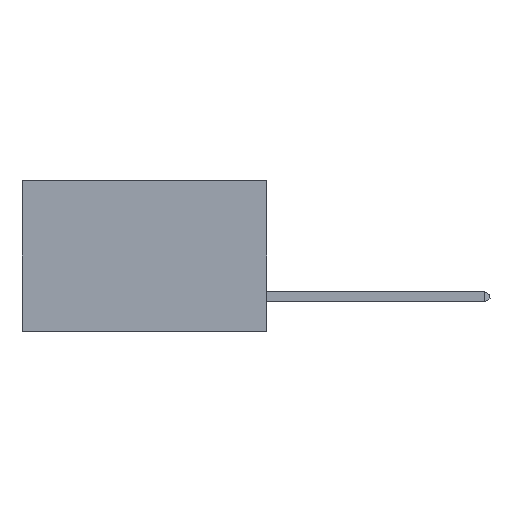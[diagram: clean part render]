
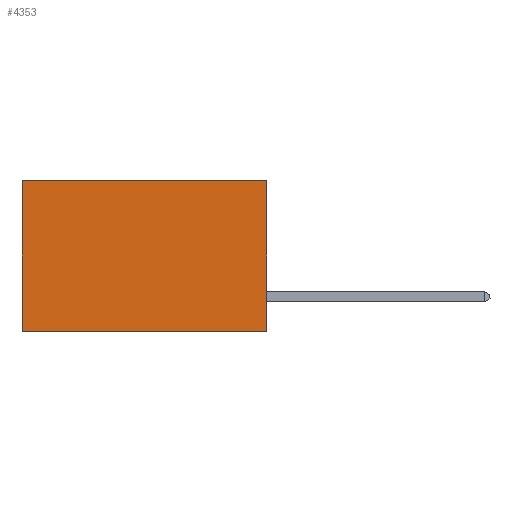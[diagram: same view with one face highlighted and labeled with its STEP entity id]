
A CAD part, left-side view. The second image highlights one B-rep face of the part: STEP entity #4353.
In plain terms, the highlighted planar face has unit normal (-1, 0, 0).
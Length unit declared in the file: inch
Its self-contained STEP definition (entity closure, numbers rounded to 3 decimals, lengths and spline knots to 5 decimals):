
#1136 = CARTESIAN_POINT ( 'NONE',  ( 0.2875, 0., 0. ) ) ;
#2256 = CARTESIAN_POINT ( 'NONE',  ( 0.2875, 0., 0. ) ) ;
#3129 = LINE ( 'NONE', #4401, #30596 ) ;
#3956 = LINE ( 'NONE', #25952, #26061 ) ;
#4353 = ADVANCED_FACE ( 'NONE', ( #4934 ), #23430, .F. ) ;
#4401 = CARTESIAN_POINT ( 'NONE',  ( 0.2875, 0., -0.37 ) ) ;
#4934 = FACE_OUTER_BOUND ( 'NONE', #14066, .T. ) ;
#5950 = DIRECTION ( 'NONE',  ( 1., 0., 0. ) ) ;
#6538 = DIRECTION ( 'NONE',  ( 0., 0., -1. ) ) ;
#8225 = EDGE_CURVE ( 'NONE', #13821, #19185, #3956, .T. ) ;
#9871 = VERTEX_POINT ( 'NONE', #10964 ) ;
#10056 = VERTEX_POINT ( 'NONE', #30152 ) ;
#10964 = CARTESIAN_POINT ( 'NONE',  ( 0.2875, 0., -0.37 ) ) ;
#11171 = VECTOR ( 'NONE', #6538, 39.37008 ) ;
#11800 = AXIS2_PLACEMENT_3D ( 'NONE', #29299, #5950, #22975 ) ;
#12745 = VECTOR ( 'NONE', #18794, 39.37008 ) ;
#13821 = VERTEX_POINT ( 'NONE', #2256 ) ;
#14066 = EDGE_LOOP ( 'NONE', ( #28393, #21594, #18133, #33533 ) ) ;
#16141 = CARTESIAN_POINT ( 'NONE',  ( 0.2875, 0.6, 0. ) ) ;
#18091 = DIRECTION ( 'NONE',  ( 0., 1., 0. ) ) ;
#18133 = ORIENTED_EDGE ( 'NONE', *, *, #21793, .F. ) ;
#18794 = DIRECTION ( 'NONE',  ( 0., 0., -1. ) ) ;
#19185 = VERTEX_POINT ( 'NONE', #33428 ) ;
#21594 = ORIENTED_EDGE ( 'NONE', *, *, #27763, .F. ) ;
#21793 = EDGE_CURVE ( 'NONE', #13821, #9871, #26100, .T. ) ;
#22975 = DIRECTION ( 'NONE',  ( 0., 0., -1. ) ) ;
#23430 = PLANE ( 'NONE',  #11800 ) ;
#23487 = EDGE_CURVE ( 'NONE', #19185, #10056, #33804, .T. ) ;
#25699 = DIRECTION ( 'NONE',  ( 0., 1., 0. ) ) ;
#25952 = CARTESIAN_POINT ( 'NONE',  ( 0.2875, 0., 0. ) ) ;
#26061 = VECTOR ( 'NONE', #18091, 39.37008 ) ;
#26100 = LINE ( 'NONE', #1136, #11171 ) ;
#27763 = EDGE_CURVE ( 'NONE', #9871, #10056, #3129, .T. ) ;
#28393 = ORIENTED_EDGE ( 'NONE', *, *, #23487, .T. ) ;
#29299 = CARTESIAN_POINT ( 'NONE',  ( 0.2875, 0., 0. ) ) ;
#30152 = CARTESIAN_POINT ( 'NONE',  ( 0.2875, 0.6, -0.37 ) ) ;
#30596 = VECTOR ( 'NONE', #25699, 39.37008 ) ;
#33428 = CARTESIAN_POINT ( 'NONE',  ( 0.2875, 0.6, 0. ) ) ;
#33533 = ORIENTED_EDGE ( 'NONE', *, *, #8225, .T. ) ;
#33804 = LINE ( 'NONE', #16141, #12745 ) ;
